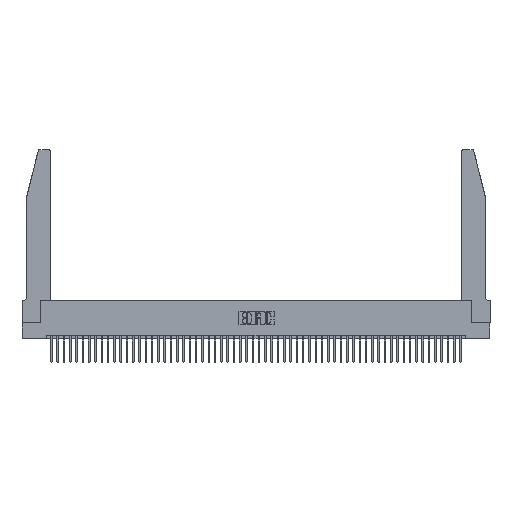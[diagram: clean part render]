
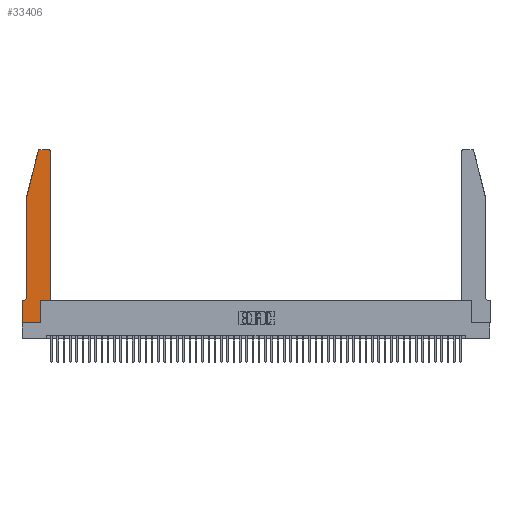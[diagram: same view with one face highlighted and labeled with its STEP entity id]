
A CAD part, top view. The second image highlights one B-rep face of the part: STEP entity #33406.
In plain terms, the highlighted planar face has unit normal (0, 0, 1).
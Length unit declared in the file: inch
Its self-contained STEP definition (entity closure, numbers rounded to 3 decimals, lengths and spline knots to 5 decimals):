
#147 = EDGE_CURVE ( 'NONE', #42591, #13304, #18983, .T. ) ;
#572 = CIRCLE ( 'NONE', #52921, 0.07 ) ;
#866 = VERTEX_POINT ( 'NONE', #33559 ) ;
#1099 = VECTOR ( 'NONE', #6708, 39.37008 ) ;
#1933 = ORIENTED_EDGE ( 'NONE', *, *, #11043, .T. ) ;
#2029 = CARTESIAN_POINT ( 'NONE',  ( 0.4205, 2.75, 0.37 ) ) ;
#2342 = CARTESIAN_POINT ( 'NONE',  ( 0.4505, 0.35, 0.37 ) ) ;
#3582 = ORIENTED_EDGE ( 'NONE', *, *, #10736, .T. ) ;
#3672 = DIRECTION ( 'NONE',  ( 0., 0., 1. ) ) ;
#3729 = CARTESIAN_POINT ( 'NONE',  ( 0.0055, 0.42, 0.37 ) ) ;
#4775 = ORIENTED_EDGE ( 'NONE', *, *, #147, .T. ) ;
#5068 = VERTEX_POINT ( 'NONE', #37220 ) ;
#5155 = VERTEX_POINT ( 'NONE', #30793 ) ;
#5862 = DIRECTION ( 'NONE',  ( 0., 0., 1. ) ) ;
#5998 = VERTEX_POINT ( 'NONE', #53283 ) ;
#6013 = DIRECTION ( 'NONE',  ( -1., 0., 0. ) ) ;
#6708 = DIRECTION ( 'NONE',  ( 0., 1., 0. ) ) ;
#7003 = CARTESIAN_POINT ( 'NONE',  ( 0.25487, 2.72718, 0.37 ) ) ;
#7109 = DIRECTION ( 'NONE',  ( 1., 0., 0. ) ) ;
#7163 = EDGE_CURVE ( 'NONE', #15326, #9158, #13386, .T. ) ;
#9158 = VERTEX_POINT ( 'NONE', #51682 ) ;
#9599 = CARTESIAN_POINT ( 'NONE',  ( 0.284, 2.72, 0.37 ) ) ;
#9783 = DIRECTION ( 'NONE',  ( -1., 0., 0. ) ) ;
#10656 = ORIENTED_EDGE ( 'NONE', *, *, #25439, .T. ) ;
#10736 = EDGE_CURVE ( 'NONE', #13304, #866, #20689, .T. ) ;
#10815 = VECTOR ( 'NONE', #42952, 39.37008 ) ;
#11043 = EDGE_CURVE ( 'NONE', #866, #15326, #28440, .T. ) ;
#11993 = VERTEX_POINT ( 'NONE', #11998 ) ;
#11998 = CARTESIAN_POINT ( 'NONE',  ( 0.0055, 0.35, 0.37 ) ) ;
#12114 = AXIS2_PLACEMENT_3D ( 'NONE', #9599, #39127, #26180 ) ;
#12233 = EDGE_CURVE ( 'NONE', #5068, #5998, #21787, .T. ) ;
#12849 = CARTESIAN_POINT ( 'NONE',  ( 0.2865, 0.35, 0.37 ) ) ;
#13304 = VERTEX_POINT ( 'NONE', #32976 ) ;
#13386 = LINE ( 'NONE', #31277, #1099 ) ;
#14316 = CARTESIAN_POINT ( 'NONE',  ( 0.0755, 2., 0.37 ) ) ;
#14634 = DIRECTION ( 'NONE',  ( 1., 0., 0. ) ) ;
#15326 = VERTEX_POINT ( 'NONE', #31972 ) ;
#16035 = FACE_OUTER_BOUND ( 'NONE', #50217, .T. ) ;
#17031 = LINE ( 'NONE', #34306, #31303 ) ;
#18351 = CARTESIAN_POINT ( 'NONE',  ( 0.4205, 2.72, 0.37 ) ) ;
#18983 = LINE ( 'NONE', #33283, #52494 ) ;
#20689 = LINE ( 'NONE', #12849, #32298 ) ;
#21230 = EDGE_CURVE ( 'NONE', #9158, #24298, #33678, .T. ) ;
#21787 = LINE ( 'NONE', #14316, #10815 ) ;
#23147 = EDGE_CURVE ( 'NONE', #5155, #42591, #52940, .T. ) ;
#24298 = VERTEX_POINT ( 'NONE', #2029 ) ;
#24626 = EDGE_CURVE ( 'NONE', #39722, #30603, #32836, .T. ) ;
#25431 = AXIS2_PLACEMENT_3D ( 'NONE', #18351, #5862, #35470 ) ;
#25439 = EDGE_CURVE ( 'NONE', #30603, #5068, #47624, .T. ) ;
#26180 = DIRECTION ( 'NONE',  ( 1., 0., 0. ) ) ;
#27125 = VECTOR ( 'NONE', #14634, 39.37008 ) ;
#28100 = DIRECTION ( 'NONE',  ( -0.239, -0.971, 0. ) ) ;
#28431 = CARTESIAN_POINT ( 'NONE',  ( 0., 0.35, 0.37 ) ) ;
#28440 = LINE ( 'NONE', #2342, #27125 ) ;
#28656 = VECTOR ( 'NONE', #6013, 39.37008 ) ;
#29526 = ORIENTED_EDGE ( 'NONE', *, *, #47308, .T. ) ;
#30491 = CARTESIAN_POINT ( 'NONE',  ( 0., 0., 0.37 ) ) ;
#30603 = VERTEX_POINT ( 'NONE', #7003 ) ;
#30793 = CARTESIAN_POINT ( 'NONE',  ( 0., 0.35, 0.37 ) ) ;
#31206 = ORIENTED_EDGE ( 'NONE', *, *, #12233, .T. ) ;
#31277 = CARTESIAN_POINT ( 'NONE',  ( 0.4505, 0.35, 0.37 ) ) ;
#31303 = VECTOR ( 'NONE', #9783, 39.37008 ) ;
#31868 = PLANE ( 'NONE',  #38643 ) ;
#31972 = CARTESIAN_POINT ( 'NONE',  ( 0.4505, 0.35, 0.37 ) ) ;
#32298 = VECTOR ( 'NONE', #37527, 39.37008 ) ;
#32508 = LINE ( 'NONE', #42801, #28656 ) ;
#32836 = CIRCLE ( 'NONE', #12114, 0.03 ) ;
#32976 = CARTESIAN_POINT ( 'NONE',  ( 0.2865, 0., 0.37 ) ) ;
#33283 = CARTESIAN_POINT ( 'NONE',  ( 0., 0., 0.37 ) ) ;
#33406 = ADVANCED_FACE ( 'NONE', ( #16035 ), #31868, .T. ) ;
#33559 = CARTESIAN_POINT ( 'NONE',  ( 0.2865, 0.35, 0.37 ) ) ;
#33678 = CIRCLE ( 'NONE', #25431, 0.03 ) ;
#34306 = CARTESIAN_POINT ( 'NONE',  ( 0.0755, 0.35, 0.37 ) ) ;
#34997 = CARTESIAN_POINT ( 'NONE',  ( 0., 0., 0.37 ) ) ;
#35470 = DIRECTION ( 'NONE',  ( 1., 0., 0. ) ) ;
#36014 = VECTOR ( 'NONE', #28100, 39.37008 ) ;
#36080 = ORIENTED_EDGE ( 'NONE', *, *, #21230, .T. ) ;
#37220 = CARTESIAN_POINT ( 'NONE',  ( 0.0755, 2., 0.37 ) ) ;
#37527 = DIRECTION ( 'NONE',  ( 0., 1., 0. ) ) ;
#38643 = AXIS2_PLACEMENT_3D ( 'NONE', #28431, #3672, #7109 ) ;
#39127 = DIRECTION ( 'NONE',  ( 0., 0., 1. ) ) ;
#39722 = VERTEX_POINT ( 'NONE', #53322 ) ;
#41053 = DIRECTION ( 'NONE',  ( -1., 0., 0. ) ) ;
#41232 = ORIENTED_EDGE ( 'NONE', *, *, #24626, .T. ) ;
#41766 = ORIENTED_EDGE ( 'NONE', *, *, #23147, .T. ) ;
#42591 = VERTEX_POINT ( 'NONE', #34997 ) ;
#42801 = CARTESIAN_POINT ( 'NONE',  ( 0.2605, 2.75, 0.37 ) ) ;
#42952 = DIRECTION ( 'NONE',  ( 0., -1., 0. ) ) ;
#44645 = ORIENTED_EDGE ( 'NONE', *, *, #49782, .T. ) ;
#44839 = DIRECTION ( 'NONE',  ( 0., 0., -1. ) ) ;
#44994 = CARTESIAN_POINT ( 'NONE',  ( 0.0755, 2., 0.37 ) ) ;
#45157 = DIRECTION ( 'NONE',  ( 1., 0., 0. ) ) ;
#46104 = EDGE_CURVE ( 'NONE', #11993, #5155, #17031, .T. ) ;
#47308 = EDGE_CURVE ( 'NONE', #24298, #39722, #32508, .T. ) ;
#47624 = LINE ( 'NONE', #44994, #36014 ) ;
#47807 = VECTOR ( 'NONE', #51277, 39.37008 ) ;
#49782 = EDGE_CURVE ( 'NONE', #5998, #11993, #572, .T. ) ;
#49798 = ORIENTED_EDGE ( 'NONE', *, *, #46104, .T. ) ;
#50217 = EDGE_LOOP ( 'NONE', ( #29526, #41232, #10656, #31206, #44645, #49798, #41766, #4775, #3582, #1933, #53104, #36080 ) ) ;
#51277 = DIRECTION ( 'NONE',  ( 0., -1., 0. ) ) ;
#51682 = CARTESIAN_POINT ( 'NONE',  ( 0.4505, 2.72, 0.37 ) ) ;
#52494 = VECTOR ( 'NONE', #45157, 39.37008 ) ;
#52921 = AXIS2_PLACEMENT_3D ( 'NONE', #3729, #44839, #41053 ) ;
#52940 = LINE ( 'NONE', #30491, #47807 ) ;
#53104 = ORIENTED_EDGE ( 'NONE', *, *, #7163, .T. ) ;
#53283 = CARTESIAN_POINT ( 'NONE',  ( 0.0755, 0.42, 0.37 ) ) ;
#53322 = CARTESIAN_POINT ( 'NONE',  ( 0.284, 2.75, 0.37 ) ) ;
